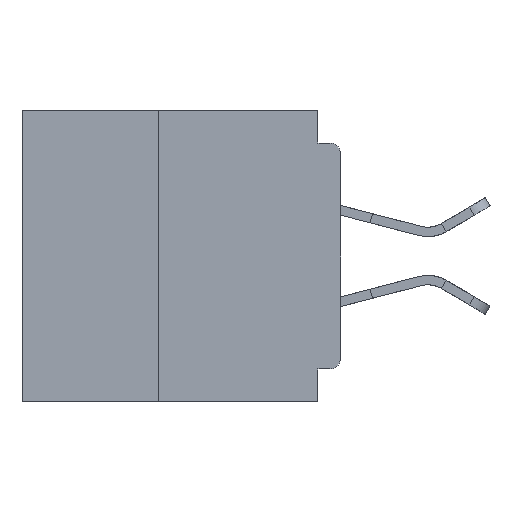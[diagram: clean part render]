
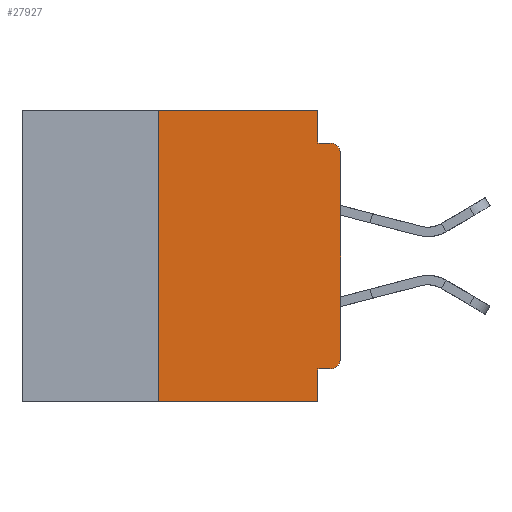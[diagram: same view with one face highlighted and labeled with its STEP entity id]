
A CAD part, left-side view. The second image highlights one B-rep face of the part: STEP entity #27927.
In plain terms, the highlighted planar face has unit normal (-1, 0, 0).
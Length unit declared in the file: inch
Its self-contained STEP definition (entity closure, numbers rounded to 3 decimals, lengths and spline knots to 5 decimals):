
#29 = CARTESIAN_POINT ( 'NONE',  ( 0., 0.437, 0. ) ) ;
#283 = CARTESIAN_POINT ( 'NONE',  ( 0., 0.25, -0.4 ) ) ;
#442 = DIRECTION ( 'NONE',  ( 0., 0., 1. ) ) ;
#1070 = VECTOR ( 'NONE', #25930, 39.37008 ) ;
#1128 = AXIS2_PLACEMENT_3D ( 'NONE', #12009, #19519, #44459 ) ;
#1351 = VERTEX_POINT ( 'NONE', #28978 ) ;
#1751 = VECTOR ( 'NONE', #38465, 39.37008 ) ;
#1882 = VERTEX_POINT ( 'NONE', #44734 ) ;
#2128 = EDGE_CURVE ( 'NONE', #1882, #12988, #34944, .T. ) ;
#2255 = CARTESIAN_POINT ( 'NONE',  ( 0., 0.031, 0. ) ) ;
#2566 = CARTESIAN_POINT ( 'NONE',  ( 0., 0., -0.06 ) ) ;
#4862 = CIRCLE ( 'NONE', #22891, 0.015 ) ;
#5229 = VERTEX_POINT ( 'NONE', #23316 ) ;
#5923 = VERTEX_POINT ( 'NONE', #13065 ) ;
#6755 = CARTESIAN_POINT ( 'NONE',  ( 0., 0.437, -0.4 ) ) ;
#6968 = ORIENTED_EDGE ( 'NONE', *, *, #2128, .T. ) ;
#7130 = VERTEX_POINT ( 'NONE', #2566 ) ;
#7557 = EDGE_CURVE ( 'NONE', #1351, #31689, #39219, .T. ) ;
#7560 = EDGE_CURVE ( 'NONE', #41843, #5229, #29775, .T. ) ;
#8000 = VECTOR ( 'NONE', #442, 39.37008 ) ;
#9140 = VERTEX_POINT ( 'NONE', #27376 ) ;
#9302 = EDGE_CURVE ( 'NONE', #13207, #5229, #23418, .T. ) ;
#10180 = ORIENTED_EDGE ( 'NONE', *, *, #9302, .T. ) ;
#10189 = CARTESIAN_POINT ( 'NONE',  ( 0., 0.015, -0.06 ) ) ;
#10251 = DIRECTION ( 'NONE',  ( 0., -1., 0. ) ) ;
#10666 = VECTOR ( 'NONE', #27420, 39.37008 ) ;
#11603 = ORIENTED_EDGE ( 'NONE', *, *, #45894, .F. ) ;
#12009 = CARTESIAN_POINT ( 'NONE',  ( 0., 0.437, 0. ) ) ;
#12035 = EDGE_CURVE ( 'NONE', #12988, #7130, #20867, .T. ) ;
#12372 = CARTESIAN_POINT ( 'NONE',  ( 0., 0., -0.355 ) ) ;
#12988 = VERTEX_POINT ( 'NONE', #36087 ) ;
#13065 = CARTESIAN_POINT ( 'NONE',  ( 0., 0.031, -0.045 ) ) ;
#13207 = VERTEX_POINT ( 'NONE', #44533 ) ;
#13824 = DIRECTION ( 'NONE',  ( 0., 0., -1. ) ) ;
#14219 = AXIS2_PLACEMENT_3D ( 'NONE', #24262, #24063, #23851 ) ;
#14998 = VECTOR ( 'NONE', #10251, 39.37008 ) ;
#15831 = FACE_OUTER_BOUND ( 'NONE', #32635, .T. ) ;
#16351 = CARTESIAN_POINT ( 'NONE',  ( 0., 0.031, 0. ) ) ;
#16536 = EDGE_CURVE ( 'NONE', #1882, #41843, #29441, .T. ) ;
#18372 = VECTOR ( 'NONE', #21611, 39.37008 ) ;
#19519 = DIRECTION ( 'NONE',  ( 1., 0., 0. ) ) ;
#19872 = VECTOR ( 'NONE', #37583, 39.37008 ) ;
#19934 = ORIENTED_EDGE ( 'NONE', *, *, #30589, .T. ) ;
#20207 = VECTOR ( 'NONE', #22316, 39.37008 ) ;
#20217 = LINE ( 'NONE', #2255, #10666 ) ;
#20519 = CARTESIAN_POINT ( 'NONE',  ( 0., 0.031, -0.355 ) ) ;
#20867 = LINE ( 'NONE', #27704, #1751 ) ;
#21611 = DIRECTION ( 'NONE',  ( 0., -1., 0. ) ) ;
#22092 = ORIENTED_EDGE ( 'NONE', *, *, #23759, .F. ) ;
#22316 = DIRECTION ( 'NONE',  ( 0., -1., 0. ) ) ;
#22891 = AXIS2_PLACEMENT_3D ( 'NONE', #10189, #35302, #13824 ) ;
#23316 = CARTESIAN_POINT ( 'NONE',  ( 0., 0.031, -0.4 ) ) ;
#23418 = LINE ( 'NONE', #6755, #14998 ) ;
#23759 = EDGE_CURVE ( 'NONE', #31689, #5923, #20217, .T. ) ;
#23851 = DIRECTION ( 'NONE',  ( 0., 0., -1. ) ) ;
#24063 = DIRECTION ( 'NONE',  ( -1., 0., 0. ) ) ;
#24262 = CARTESIAN_POINT ( 'NONE',  ( 0., 0.015, -0.34 ) ) ;
#25566 = ORIENTED_EDGE ( 'NONE', *, *, #12035, .T. ) ;
#25930 = DIRECTION ( 'NONE',  ( 0., 0., -1. ) ) ;
#27376 = CARTESIAN_POINT ( 'NONE',  ( 0., 0.015, -0.045 ) ) ;
#27420 = DIRECTION ( 'NONE',  ( 0., 0., -1. ) ) ;
#27704 = CARTESIAN_POINT ( 'NONE',  ( 0., 0., 0. ) ) ;
#27927 = ADVANCED_FACE ( 'NONE', ( #15831 ), #40899, .F. ) ;
#28978 = CARTESIAN_POINT ( 'NONE',  ( 0., 0.25, 0. ) ) ;
#29441 = LINE ( 'NONE', #12372, #19872 ) ;
#29775 = LINE ( 'NONE', #33620, #1070 ) ;
#30589 = EDGE_CURVE ( 'NONE', #7130, #9140, #4862, .T. ) ;
#30742 = ORIENTED_EDGE ( 'NONE', *, *, #32397, .F. ) ;
#31588 = ORIENTED_EDGE ( 'NONE', *, *, #7560, .F. ) ;
#31689 = VERTEX_POINT ( 'NONE', #16351 ) ;
#32397 = EDGE_CURVE ( 'NONE', #5923, #9140, #45688, .T. ) ;
#32635 = EDGE_LOOP ( 'NONE', ( #25566, #19934, #30742, #22092, #34455, #11603, #10180, #31588, #33627, #6968 ) ) ;
#33620 = CARTESIAN_POINT ( 'NONE',  ( 0., 0.031, -0.4 ) ) ;
#33627 = ORIENTED_EDGE ( 'NONE', *, *, #16536, .F. ) ;
#34455 = ORIENTED_EDGE ( 'NONE', *, *, #7557, .F. ) ;
#34944 = CIRCLE ( 'NONE', #14219, 0.015 ) ;
#35302 = DIRECTION ( 'NONE',  ( -1., 0., 0. ) ) ;
#36087 = CARTESIAN_POINT ( 'NONE',  ( 0., 0., -0.34 ) ) ;
#36663 = LINE ( 'NONE', #283, #8000 ) ;
#37583 = DIRECTION ( 'NONE',  ( 0., 1., 0. ) ) ;
#38465 = DIRECTION ( 'NONE',  ( 0., 0., 1. ) ) ;
#39219 = LINE ( 'NONE', #29, #20207 ) ;
#40899 = PLANE ( 'NONE',  #1128 ) ;
#41843 = VERTEX_POINT ( 'NONE', #20519 ) ;
#42967 = CARTESIAN_POINT ( 'NONE',  ( 0., 0., -0.045 ) ) ;
#44459 = DIRECTION ( 'NONE',  ( 0., 0., -1. ) ) ;
#44533 = CARTESIAN_POINT ( 'NONE',  ( 0., 0.25, -0.4 ) ) ;
#44734 = CARTESIAN_POINT ( 'NONE',  ( 0., 0.015, -0.355 ) ) ;
#45688 = LINE ( 'NONE', #42967, #18372 ) ;
#45894 = EDGE_CURVE ( 'NONE', #13207, #1351, #36663, .T. ) ;
